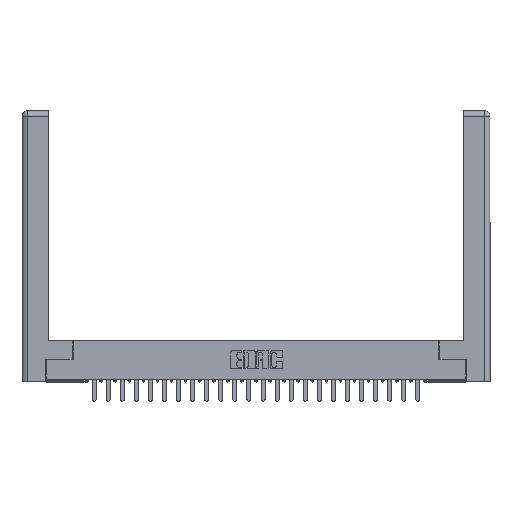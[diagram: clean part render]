
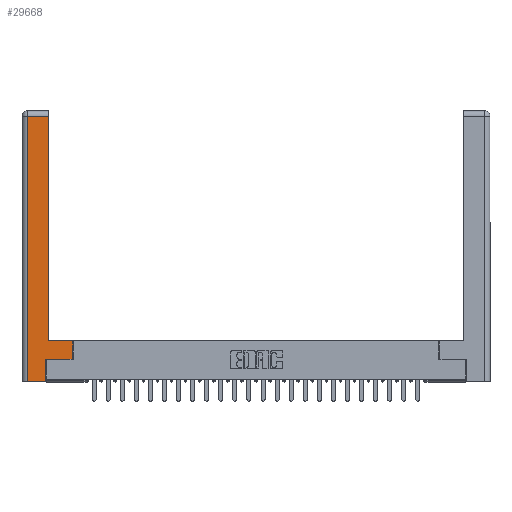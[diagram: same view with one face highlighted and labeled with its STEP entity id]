
A CAD part, top view. The second image highlights one B-rep face of the part: STEP entity #29668.
In plain terms, the highlighted planar face has unit normal (0, 0, 1).
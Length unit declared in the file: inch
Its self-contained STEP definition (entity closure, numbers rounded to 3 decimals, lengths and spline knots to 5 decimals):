
#798 = EDGE_CURVE ( 'NONE', #23553, #13764, #6720, .T. ) ;
#1442 = VECTOR ( 'NONE', #4428, 39.37008 ) ;
#2261 = DIRECTION ( 'NONE',  ( -1., 0., 0. ) ) ;
#2514 = EDGE_CURVE ( 'NONE', #13764, #13910, #20778, .T. ) ;
#2670 = EDGE_CURVE ( 'NONE', #20087, #23553, #3368, .T. ) ;
#3368 = LINE ( 'NONE', #15619, #14861 ) ;
#3481 = VERTEX_POINT ( 'NONE', #30582 ) ;
#4428 = DIRECTION ( 'NONE',  ( -1., 0., 0. ) ) ;
#4708 = CARTESIAN_POINT ( 'NONE',  ( 0.565, 0.45, 0. ) ) ;
#4878 = VECTOR ( 'NONE', #27670, 39.37008 ) ;
#5351 = DIRECTION ( 'NONE',  ( 0., -1., 0. ) ) ;
#5659 = ORIENTED_EDGE ( 'NONE', *, *, #25971, .T. ) ;
#6165 = LINE ( 'NONE', #21711, #9144 ) ;
#6293 = DIRECTION ( 'NONE',  ( 0., 1., 0. ) ) ;
#6720 = LINE ( 'NONE', #16700, #7467 ) ;
#6846 = CARTESIAN_POINT ( 'NONE',  ( 0.565, 0.45, 0. ) ) ;
#7467 = VECTOR ( 'NONE', #23740, 39.37008 ) ;
#8201 = EDGE_CURVE ( 'NONE', #3481, #8593, #30484, .T. ) ;
#8399 = AXIS2_PLACEMENT_3D ( 'NONE', #11485, #17693, #16536 ) ;
#8593 = VERTEX_POINT ( 'NONE', #21307 ) ;
#8623 = EDGE_CURVE ( 'NONE', #8593, #25384, #10359, .T. ) ;
#9144 = VECTOR ( 'NONE', #10043, 39.37008 ) ;
#9271 = VECTOR ( 'NONE', #11829, 39.37008 ) ;
#9445 = ORIENTED_EDGE ( 'NONE', *, *, #8201, .T. ) ;
#10043 = DIRECTION ( 'NONE',  ( 1., 0., 0. ) ) ;
#10359 = LINE ( 'NONE', #30365, #1442 ) ;
#11245 = CARTESIAN_POINT ( 'NONE',  ( 0.295, 3., 0. ) ) ;
#11431 = ORIENTED_EDGE ( 'NONE', *, *, #25112, .T. ) ;
#11485 = CARTESIAN_POINT ( 'NONE',  ( 0., 0., 0. ) ) ;
#11829 = DIRECTION ( 'NONE',  ( 0., 1., 0. ) ) ;
#13046 = EDGE_CURVE ( 'NONE', #25384, #25061, #24494, .T. ) ;
#13750 = VECTOR ( 'NONE', #5351, 39.37008 ) ;
#13764 = VERTEX_POINT ( 'NONE', #17955 ) ;
#13910 = VERTEX_POINT ( 'NONE', #4708 ) ;
#14861 = VECTOR ( 'NONE', #6293, 39.37008 ) ;
#14930 = CARTESIAN_POINT ( 'NONE',  ( 0.0615, 0., 0. ) ) ;
#15619 = CARTESIAN_POINT ( 'NONE',  ( 0.265, 0.245, 0. ) ) ;
#16117 = ORIENTED_EDGE ( 'NONE', *, *, #2514, .T. ) ;
#16481 = EDGE_LOOP ( 'NONE', ( #9445, #24298, #22815, #5659, #20558, #23438, #16117, #11431 ) ) ;
#16536 = DIRECTION ( 'NONE',  ( -1., 0., 0. ) ) ;
#16700 = CARTESIAN_POINT ( 'NONE',  ( 0.565, 0.245, 0. ) ) ;
#17693 = DIRECTION ( 'NONE',  ( 0., 0., -1. ) ) ;
#17955 = CARTESIAN_POINT ( 'NONE',  ( 0.565, 0.245, 0. ) ) ;
#18277 = FACE_OUTER_BOUND ( 'NONE', #16481, .T. ) ;
#19597 = LINE ( 'NONE', #26272, #21050 ) ;
#19795 = CARTESIAN_POINT ( 'NONE',  ( 0.0615, 2.94, 0. ) ) ;
#20087 = VERTEX_POINT ( 'NONE', #20492 ) ;
#20492 = CARTESIAN_POINT ( 'NONE',  ( 0.265, 0., 0. ) ) ;
#20558 = ORIENTED_EDGE ( 'NONE', *, *, #2670, .T. ) ;
#20778 = LINE ( 'NONE', #6846, #9271 ) ;
#21050 = VECTOR ( 'NONE', #2261, 39.37008 ) ;
#21307 = CARTESIAN_POINT ( 'NONE',  ( 0.295, 2.94, 0. ) ) ;
#21711 = CARTESIAN_POINT ( 'NONE',  ( 0.265, 0., 0. ) ) ;
#22815 = ORIENTED_EDGE ( 'NONE', *, *, #13046, .T. ) ;
#23438 = ORIENTED_EDGE ( 'NONE', *, *, #798, .T. ) ;
#23553 = VERTEX_POINT ( 'NONE', #27273 ) ;
#23740 = DIRECTION ( 'NONE',  ( 1., 0., 0. ) ) ;
#23912 = CARTESIAN_POINT ( 'NONE',  ( 0.0615, 0., 0. ) ) ;
#24298 = ORIENTED_EDGE ( 'NONE', *, *, #8623, .T. ) ;
#24494 = LINE ( 'NONE', #14930, #13750 ) ;
#25061 = VERTEX_POINT ( 'NONE', #23912 ) ;
#25112 = EDGE_CURVE ( 'NONE', #13910, #3481, #19597, .T. ) ;
#25384 = VERTEX_POINT ( 'NONE', #19795 ) ;
#25971 = EDGE_CURVE ( 'NONE', #25061, #20087, #6165, .T. ) ;
#26272 = CARTESIAN_POINT ( 'NONE',  ( 0.295, 0.45, 0. ) ) ;
#27273 = CARTESIAN_POINT ( 'NONE',  ( 0.265, 0.245, 0. ) ) ;
#27670 = DIRECTION ( 'NONE',  ( 0., 1., 0. ) ) ;
#29668 = ADVANCED_FACE ( 'NONE', ( #18277 ), #30422, .F. ) ;
#30365 = CARTESIAN_POINT ( 'NONE',  ( 0.0615, 2.94, 0. ) ) ;
#30422 = PLANE ( 'NONE',  #8399 ) ;
#30484 = LINE ( 'NONE', #11245, #4878 ) ;
#30582 = CARTESIAN_POINT ( 'NONE',  ( 0.295, 0.45, 0. ) ) ;
